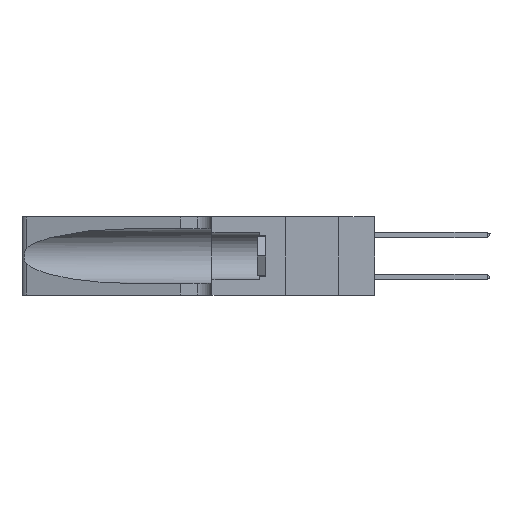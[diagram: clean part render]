
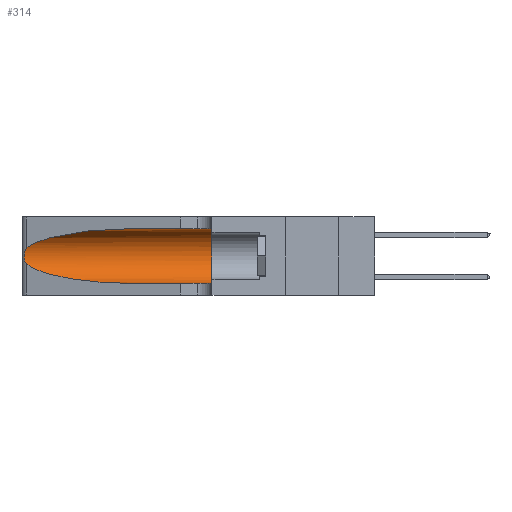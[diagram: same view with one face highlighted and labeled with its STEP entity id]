
A CAD part, left-side view. The second image highlights one B-rep face of the part: STEP entity #314.
In plain terms, the highlighted cylindrical face has radius 3.308 mm (diameter 6.617 mm), a partial arc.
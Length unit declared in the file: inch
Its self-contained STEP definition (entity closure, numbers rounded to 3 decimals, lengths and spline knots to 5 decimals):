
#314 = ADVANCED_FACE ( 'NONE', ( #36398 ), #10688, .F. ) ;
#517 = EDGE_CURVE ( 'NONE', #22878, #14523, #18631, .T. ) ;
#650 = CARTESIAN_POINT ( 'NONE',  ( 0.25487, 1.22718, 0.22369 ) ) ;
#1094 = CARTESIAN_POINT ( 'NONE',  ( 0.1305, 0.35, 0.185 ) ) ;
#1230 = DIRECTION ( 'NONE',  ( 0., 1., 0. ) ) ;
#1390 = VERTEX_POINT ( 'NONE', #29953 ) ;
#4443 = CARTESIAN_POINT ( 'NONE',  ( 0.25487, 1.22718, 0.22369 ) ) ;
#4804 = CARTESIAN_POINT ( 'NONE',  ( 0.25639, 1.23186, 0.15144 ) ) ;
#5229 = CARTESIAN_POINT ( 'NONE',  ( 0.25854, 1.2359, 0.20912 ) ) ;
#7487 = EDGE_LOOP ( 'NONE', ( #31477, #33170, #27358, #26324, #9371, #17730 ) ) ;
#7664 = CARTESIAN_POINT ( 'NONE',  ( 0.25789, 1.23486, 0.15765 ) ) ;
#8592 = CARTESIAN_POINT ( 'NONE',  ( 0.25856, 1.23593, 0.16098 ) ) ;
#9349 = EDGE_CURVE ( 'NONE', #1390, #33882, #10256, .T. ) ;
#9371 = ORIENTED_EDGE ( 'NONE', *, *, #33485, .F. ) ;
#10256 =( BOUNDED_CURVE ( )  B_SPLINE_CURVE ( 3, ( #16474, #22586, #13708, #4443 ),
 .UNSPECIFIED., .F., .F. ) 
 B_SPLINE_CURVE_WITH_KNOTS ( ( 4, 4 ),
 ( 1.5708, 2.84003 ),
 .UNSPECIFIED. ) 
 CURVE ( )  GEOMETRIC_REPRESENTATION_ITEM ( )  RATIONAL_B_SPLINE_CURVE ( ( 1., 0.87, 0.87, 1. ) ) 
 REPRESENTATION_ITEM ( '' )  );
#10688 = CYLINDRICAL_SURFACE ( 'NONE', #15410, 0.13025 ) ;
#12180 = CIRCLE ( 'NONE', #28833, 0.13025 ) ;
#12193 = CARTESIAN_POINT ( 'NONE',  ( 0.1305, 0.72297, 0.05475 ) ) ;
#12730 = CARTESIAN_POINT ( 'NONE',  ( 0.1305, 1.61858, 0.185 ) ) ;
#13011 = DIRECTION ( 'NONE',  ( 0., 0., 1. ) ) ;
#13268 = DIRECTION ( 'NONE',  ( 0., -1., 0. ) ) ;
#13643 = DIRECTION ( 'NONE',  ( 0., -1., 0. ) ) ;
#13690 = CARTESIAN_POINT ( 'NONE',  ( 0.26018, 1.23835, 0.19895 ) ) ;
#13708 = CARTESIAN_POINT ( 'NONE',  ( 0.2373, 1.15595, 0.28018 ) ) ;
#13817 = CARTESIAN_POINT ( 'NONE',  ( 0.26075, 1.23896, 0.178 ) ) ;
#14523 = VERTEX_POINT ( 'NONE', #37559 ) ;
#14785 = LINE ( 'NONE', #32023, #18007 ) ;
#15410 = AXIS2_PLACEMENT_3D ( 'NONE', #12730, #15758, #36603 ) ;
#15758 = DIRECTION ( 'NONE',  ( 0., -1., 0. ) ) ;
#16474 = CARTESIAN_POINT ( 'NONE',  ( 0.1305, 0.72297, 0.31525 ) ) ;
#16847 = CARTESIAN_POINT ( 'NONE',  ( 0.25555, 1.22994, 0.2215 ) ) ;
#17730 = ORIENTED_EDGE ( 'NONE', *, *, #21798, .F. ) ;
#18007 = VECTOR ( 'NONE', #13268, 39.37008 ) ;
#18409 = CARTESIAN_POINT ( 'NONE',  ( 0.1305, 0.72297, 0.05475 ) ) ;
#18631 = LINE ( 'NONE', #19529, #20531 ) ;
#18712 = EDGE_CURVE ( 'NONE', #33882, #24092, #37311, .T. ) ;
#19529 = CARTESIAN_POINT ( 'NONE',  ( 0.1305, 1.61858, 0.05475 ) ) ;
#19588 = CARTESIAN_POINT ( 'NONE',  ( 0.25639, 1.23184, 0.21858 ) ) ;
#19971 = CARTESIAN_POINT ( 'NONE',  ( 0.25787, 1.23484, 0.2124 ) ) ;
#20331 = CARTESIAN_POINT ( 'NONE',  ( 0.2373, 1.15595, 0.08982 ) ) ;
#20531 = VECTOR ( 'NONE', #13643, 39.37008 ) ;
#21798 = EDGE_CURVE ( 'NONE', #1390, #27828, #14785, .T. ) ;
#22586 = CARTESIAN_POINT ( 'NONE',  ( 0.18966, 0.96281, 0.31525 ) ) ;
#22878 = VERTEX_POINT ( 'NONE', #18409 ) ;
#23269 = CARTESIAN_POINT ( 'NONE',  ( 0.25487, 1.22718, 0.14631 ) ) ;
#24092 = VERTEX_POINT ( 'NONE', #24477 ) ;
#24477 = CARTESIAN_POINT ( 'NONE',  ( 0.25487, 1.22718, 0.14631 ) ) ;
#25449 = CARTESIAN_POINT ( 'NONE',  ( 0.25555, 1.22993, 0.14849 ) ) ;
#25538 = CARTESIAN_POINT ( 'NONE',  ( 0.25487, 1.22718, 0.22369 ) ) ;
#26324 = ORIENTED_EDGE ( 'NONE', *, *, #517, .T. ) ;
#27358 = ORIENTED_EDGE ( 'NONE', *, *, #29774, .T. ) ;
#27828 = VERTEX_POINT ( 'NONE', #32520 ) ;
#28674 = CARTESIAN_POINT ( 'NONE',  ( 0.26075, 1.23896, 0.19203 ) ) ;
#28833 = AXIS2_PLACEMENT_3D ( 'NONE', #1094, #1230, #13011 ) ;
#29774 = EDGE_CURVE ( 'NONE', #24092, #22878, #31548, .T. ) ;
#29837 = CARTESIAN_POINT ( 'NONE',  ( 0.18966, 0.96281, 0.05475 ) ) ;
#29953 = CARTESIAN_POINT ( 'NONE',  ( 0.1305, 0.72297, 0.31525 ) ) ;
#31477 = ORIENTED_EDGE ( 'NONE', *, *, #9349, .T. ) ;
#31548 =( BOUNDED_CURVE ( )  B_SPLINE_CURVE ( 3, ( #32157, #20331, #29837, #12193 ),
 .UNSPECIFIED., .F., .F. ) 
 B_SPLINE_CURVE_WITH_KNOTS ( ( 4, 4 ),
 ( 3.44316, 4.71239 ),
 .UNSPECIFIED. ) 
 CURVE ( )  GEOMETRIC_REPRESENTATION_ITEM ( )  RATIONAL_B_SPLINE_CURVE ( ( 1., 0.87, 0.87, 1. ) ) 
 REPRESENTATION_ITEM ( '' )  );
#32023 = CARTESIAN_POINT ( 'NONE',  ( 0.1305, 1.61858, 0.31525 ) ) ;
#32157 = CARTESIAN_POINT ( 'NONE',  ( 0.25487, 1.22718, 0.14631 ) ) ;
#32520 = CARTESIAN_POINT ( 'NONE',  ( 0.1305, 0.35, 0.31525 ) ) ;
#33170 = ORIENTED_EDGE ( 'NONE', *, *, #18712, .T. ) ;
#33485 = EDGE_CURVE ( 'NONE', #27828, #14523, #12180, .T. ) ;
#33882 = VERTEX_POINT ( 'NONE', #650 ) ;
#34697 = CARTESIAN_POINT ( 'NONE',  ( 0.26017, 1.23833, 0.17102 ) ) ;
#36398 = FACE_OUTER_BOUND ( 'NONE', #7487, .T. ) ;
#36603 = DIRECTION ( 'NONE',  ( 0., 0., -1. ) ) ;
#37311 = B_SPLINE_CURVE_WITH_KNOTS ( 'NONE', 3,
 ( #25538, #16847, #19588, #19971, #5229, #13690, #28674, #13817, #34697, #8592, #7664, #4804, #25449, #23269 ),
 .UNSPECIFIED., .F., .F.,
 ( 4, 2, 2, 2, 2, 2, 4 ),
 ( 0., 0.00027, 0.00053, 0.00107, 0.0016, 0.00187, 0.00214 ),
 .UNSPECIFIED. ) ;
#37559 = CARTESIAN_POINT ( 'NONE',  ( 0.1305, 0.35, 0.05475 ) ) ;
